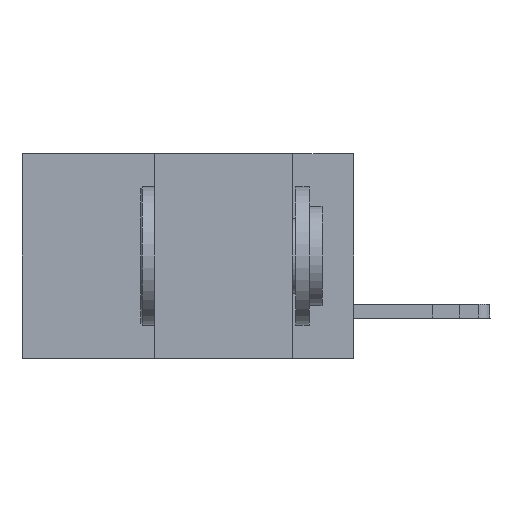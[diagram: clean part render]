
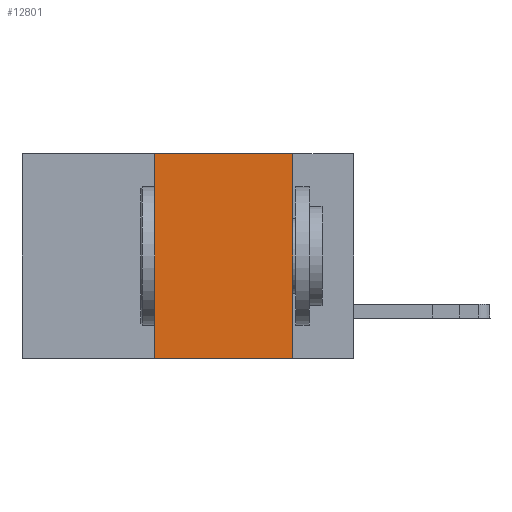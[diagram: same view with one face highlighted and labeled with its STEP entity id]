
A CAD part, left-side view. The second image highlights one B-rep face of the part: STEP entity #12801.
In plain terms, the highlighted planar face has unit normal (-1, 0, 0).
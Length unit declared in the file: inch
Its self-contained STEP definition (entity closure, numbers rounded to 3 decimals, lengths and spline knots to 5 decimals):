
#1819 = LINE ( 'NONE', #7964, #10368 ) ;
#2001 = CARTESIAN_POINT ( 'NONE',  ( 0., 0.36, -0.37 ) ) ;
#2446 = ORIENTED_EDGE ( 'NONE', *, *, #6375, .F. ) ;
#2839 = DIRECTION ( 'NONE',  ( 0., 0., -1. ) ) ;
#3062 = VERTEX_POINT ( 'NONE', #15298 ) ;
#3508 = ORIENTED_EDGE ( 'NONE', *, *, #14213, .F. ) ;
#5434 = AXIS2_PLACEMENT_3D ( 'NONE', #8472, #20126, #10156 ) ;
#6199 = CARTESIAN_POINT ( 'NONE',  ( 0., 0.36, 0. ) ) ;
#6375 = EDGE_CURVE ( 'NONE', #19949, #3062, #1819, .T. ) ;
#7709 = LINE ( 'NONE', #21499, #20450 ) ;
#7964 = CARTESIAN_POINT ( 'NONE',  ( 0., 0.11, 0. ) ) ;
#8472 = CARTESIAN_POINT ( 'NONE',  ( 0., 0.6, 0. ) ) ;
#9574 = DIRECTION ( 'NONE',  ( 0., 0., 1. ) ) ;
#10156 = DIRECTION ( 'NONE',  ( 0., 0., -1. ) ) ;
#10368 = VECTOR ( 'NONE', #2839, 39.37008 ) ;
#10755 = FACE_OUTER_BOUND ( 'NONE', #20172, .T. ) ;
#10845 = CARTESIAN_POINT ( 'NONE',  ( 0., 0.6, -0.37 ) ) ;
#11464 = ORIENTED_EDGE ( 'NONE', *, *, #17216, .F. ) ;
#12624 = VECTOR ( 'NONE', #14169, 39.37008 ) ;
#12801 = ADVANCED_FACE ( 'NONE', ( #10755 ), #13423, .F. ) ;
#13037 = ORIENTED_EDGE ( 'NONE', *, *, #17546, .T. ) ;
#13142 = LINE ( 'NONE', #10845, #12624 ) ;
#13423 = PLANE ( 'NONE',  #5434 ) ;
#14169 = DIRECTION ( 'NONE',  ( 0., -1., 0. ) ) ;
#14213 = EDGE_CURVE ( 'NONE', #19672, #15581, #15330, .T. ) ;
#15298 = CARTESIAN_POINT ( 'NONE',  ( 0., 0.11, -0.37 ) ) ;
#15330 = LINE ( 'NONE', #6199, #15848 ) ;
#15581 = VERTEX_POINT ( 'NONE', #21568 ) ;
#15848 = VECTOR ( 'NONE', #9574, 39.37008 ) ;
#17216 = EDGE_CURVE ( 'NONE', #15581, #19949, #7709, .T. ) ;
#17546 = EDGE_CURVE ( 'NONE', #19672, #3062, #13142, .T. ) ;
#17842 = CARTESIAN_POINT ( 'NONE',  ( 0., 0.11, 0. ) ) ;
#19672 = VERTEX_POINT ( 'NONE', #2001 ) ;
#19949 = VERTEX_POINT ( 'NONE', #17842 ) ;
#20126 = DIRECTION ( 'NONE',  ( 1., 0., 0. ) ) ;
#20172 = EDGE_LOOP ( 'NONE', ( #2446, #11464, #3508, #13037 ) ) ;
#20450 = VECTOR ( 'NONE', #21433, 39.37008 ) ;
#21433 = DIRECTION ( 'NONE',  ( 0., -1., 0. ) ) ;
#21499 = CARTESIAN_POINT ( 'NONE',  ( 0., 0.6, 0. ) ) ;
#21568 = CARTESIAN_POINT ( 'NONE',  ( 0., 0.36, 0. ) ) ;
